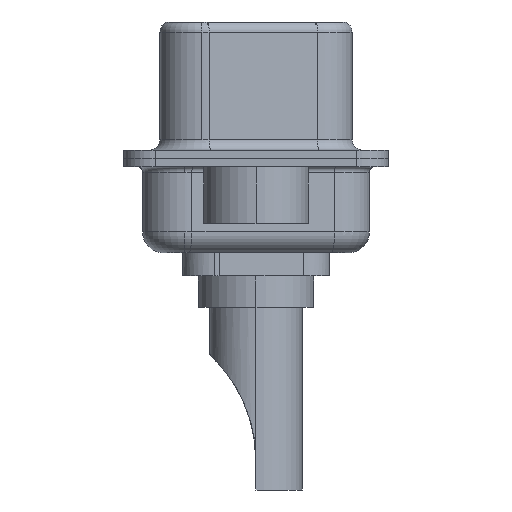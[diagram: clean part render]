
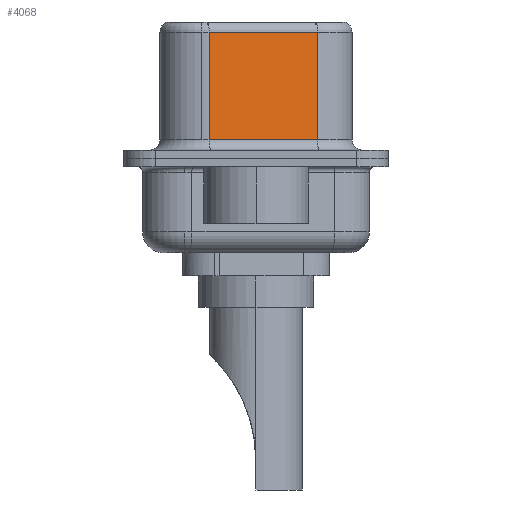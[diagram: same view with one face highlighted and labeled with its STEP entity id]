
A CAD part, left-side view. The second image highlights one B-rep face of the part: STEP entity #4068.
In plain terms, the highlighted planar face has unit normal (-0.985, -0.174, 0).
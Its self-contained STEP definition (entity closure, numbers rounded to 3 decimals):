
#961 = VERTEX_POINT ( 'NONE', #8666 ) ;
#2511 = CARTESIAN_POINT ( 'NONE',  ( 4.58, -2.927, 6.52 ) ) ;
#3477 = CARTESIAN_POINT ( 'NONE',  ( 4.58, -2.927, 6.52 ) ) ;
#3565 = VERTEX_POINT ( 'NONE', #15326 ) ;
#3611 = ORIENTED_EDGE ( 'NONE', *, *, #16667, .T. ) ;
#4068 = ADVANCED_FACE ( 'NONE', ( #10772 ), #7013, .F. ) ;
#5006 = CARTESIAN_POINT ( 'NONE',  ( 4.58, -2.927, 0.9 ) ) ;
#6923 = CARTESIAN_POINT ( 'NONE',  ( 4.58, -2.927, 6.02 ) ) ;
#7013 = PLANE ( 'NONE',  #19852 ) ;
#7093 = DIRECTION ( 'NONE',  ( 0., 0., -1. ) ) ;
#7692 = VECTOR ( 'NONE', #9432, 1000. ) ;
#7804 = ORIENTED_EDGE ( 'NONE', *, *, #18018, .F. ) ;
#8666 = CARTESIAN_POINT ( 'NONE',  ( 3.67, 2.233, 6.02 ) ) ;
#9036 = ORIENTED_EDGE ( 'NONE', *, *, #12731, .T. ) ;
#9188 = DIRECTION ( 'NONE',  ( 0.985, 0.174, 0. ) ) ;
#9330 = VECTOR ( 'NONE', #15858, 1000. ) ;
#9432 = DIRECTION ( 'NONE',  ( 0.174, -0.985, 0. ) ) ;
#9485 = LINE ( 'NONE', #22581, #13140 ) ;
#9993 = DIRECTION ( 'NONE',  ( 0., 0., -1. ) ) ;
#10772 = FACE_OUTER_BOUND ( 'NONE', #15285, .T. ) ;
#10851 = VERTEX_POINT ( 'NONE', #13139 ) ;
#12514 = LINE ( 'NONE', #18395, #7692 ) ;
#12731 = EDGE_CURVE ( 'NONE', #3565, #23573, #12514, .T. ) ;
#13139 = CARTESIAN_POINT ( 'NONE',  ( 4.58, -2.927, 6.02 ) ) ;
#13140 = VECTOR ( 'NONE', #9993, 1000. ) ;
#13220 = VECTOR ( 'NONE', #7093, 1000. ) ;
#15285 = EDGE_LOOP ( 'NONE', ( #7804, #3611, #22997, #9036 ) ) ;
#15326 = CARTESIAN_POINT ( 'NONE',  ( 3.67, 2.233, 0.9 ) ) ;
#15858 = DIRECTION ( 'NONE',  ( -0.174, 0.985, 0. ) ) ;
#16667 = EDGE_CURVE ( 'NONE', #10851, #961, #19462, .T. ) ;
#17998 = LINE ( 'NONE', #3477, #13220 ) ;
#18018 = EDGE_CURVE ( 'NONE', #10851, #23573, #17998, .T. ) ;
#18395 = CARTESIAN_POINT ( 'NONE',  ( 4.58, -2.927, 0.9 ) ) ;
#19063 = DIRECTION ( 'NONE',  ( -0.174, 0.985, 0. ) ) ;
#19462 = LINE ( 'NONE', #6923, #9330 ) ;
#19552 = EDGE_CURVE ( 'NONE', #961, #3565, #9485, .T. ) ;
#19852 = AXIS2_PLACEMENT_3D ( 'NONE', #2511, #9188, #19063 ) ;
#22581 = CARTESIAN_POINT ( 'NONE',  ( 3.67, 2.233, 6.52 ) ) ;
#22997 = ORIENTED_EDGE ( 'NONE', *, *, #19552, .T. ) ;
#23573 = VERTEX_POINT ( 'NONE', #5006 ) ;
